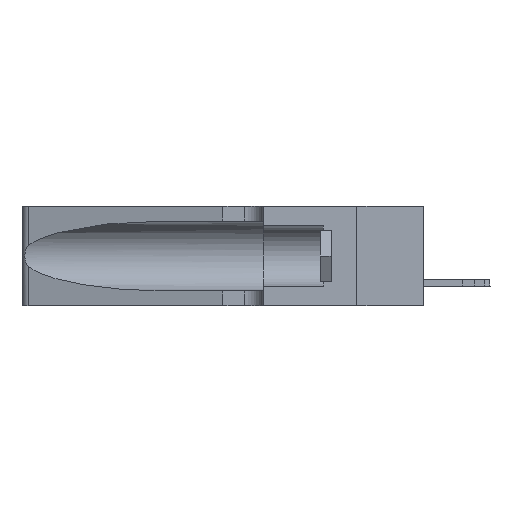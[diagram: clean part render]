
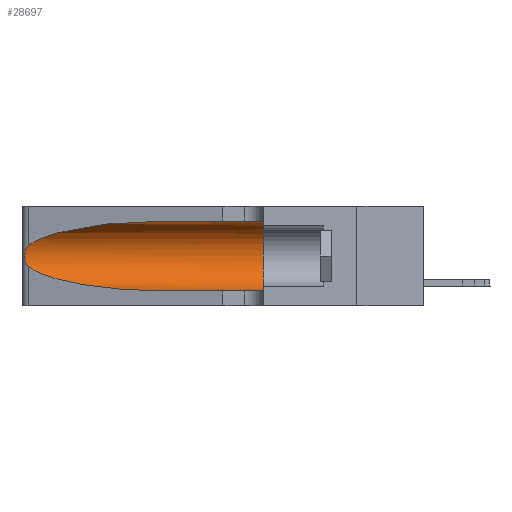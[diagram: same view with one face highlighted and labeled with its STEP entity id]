
A CAD part, left-side view. The second image highlights one B-rep face of the part: STEP entity #28697.
In plain terms, the highlighted cylindrical face has radius 3.308 mm (diameter 6.617 mm), a partial arc.
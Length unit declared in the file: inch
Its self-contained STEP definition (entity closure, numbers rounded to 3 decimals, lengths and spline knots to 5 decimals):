
#554 =( BOUNDED_CURVE ( )  B_SPLINE_CURVE ( 3, ( #15798, #22592, #4227, #18102 ),
 .UNSPECIFIED., .F., .T. ) 
 B_SPLINE_CURVE_WITH_KNOTS ( ( 4, 4 ),
 ( 3.44316, 4.71239 ),
 .UNSPECIFIED. ) 
 CURVE ( )  GEOMETRIC_REPRESENTATION_ITEM ( )  RATIONAL_B_SPLINE_CURVE ( ( 1., 0.87, 0.87, 1. ) ) 
 REPRESENTATION_ITEM ( '' )  );
#1014 = AXIS2_PLACEMENT_3D ( 'NONE', #15501, #12953, #17614 ) ;
#1427 = EDGE_LOOP ( 'NONE', ( #17655, #5297, #15512, #22694, #8040, #17215 ) ) ;
#1759 = CARTESIAN_POINT ( 'NONE',  ( 0.25639, 1.23184, 0.21858 ) ) ;
#2058 = VERTEX_POINT ( 'NONE', #29557 ) ;
#2132 = CARTESIAN_POINT ( 'NONE',  ( 0.1305, 0.72297, 0.31525 ) ) ;
#2255 = CARTESIAN_POINT ( 'NONE',  ( 0.1305, 0.72297, 0.31525 ) ) ;
#2358 = CARTESIAN_POINT ( 'NONE',  ( 0.18966, 0.96281, 0.31525 ) ) ;
#3695 = CARTESIAN_POINT ( 'NONE',  ( 0.25856, 1.23593, 0.16098 ) ) ;
#3727 = VERTEX_POINT ( 'NONE', #7228 ) ;
#3909 = CARTESIAN_POINT ( 'NONE',  ( 0.25787, 1.23484, 0.2124 ) ) ;
#3962 = VERTEX_POINT ( 'NONE', #2132 ) ;
#4227 = CARTESIAN_POINT ( 'NONE',  ( 0.18966, 0.96281, 0.05475 ) ) ;
#4810 = EDGE_CURVE ( 'NONE', #20243, #8025, #29675, .T. ) ;
#5297 = ORIENTED_EDGE ( 'NONE', *, *, #4810, .T. ) ;
#6136 = CARTESIAN_POINT ( 'NONE',  ( 0.25854, 1.2359, 0.20912 ) ) ;
#6489 = LINE ( 'NONE', #26555, #17339 ) ;
#6743 = CARTESIAN_POINT ( 'NONE',  ( 0.25487, 1.22718, 0.22369 ) ) ;
#7044 = EDGE_CURVE ( 'NONE', #26995, #2058, #26126, .T. ) ;
#7228 = CARTESIAN_POINT ( 'NONE',  ( 0.1305, 0.72297, 0.05475 ) ) ;
#8025 = VERTEX_POINT ( 'NONE', #8267 ) ;
#8040 = ORIENTED_EDGE ( 'NONE', *, *, #7044, .F. ) ;
#8267 = CARTESIAN_POINT ( 'NONE',  ( 0.25487, 1.22718, 0.14631 ) ) ;
#8480 = DIRECTION ( 'NONE',  ( 0., -1., 0. ) ) ;
#8678 = CARTESIAN_POINT ( 'NONE',  ( 0.25487, 1.22718, 0.22369 ) ) ;
#8778 = CARTESIAN_POINT ( 'NONE',  ( 0.25555, 1.22994, 0.2215 ) ) ;
#8940 = EDGE_CURVE ( 'NONE', #3727, #2058, #6489, .T. ) ;
#10435 = DIRECTION ( 'NONE',  ( 0., -1., 0. ) ) ;
#10907 = CARTESIAN_POINT ( 'NONE',  ( 0.25555, 1.22993, 0.14849 ) ) ;
#11491 = CARTESIAN_POINT ( 'NONE',  ( 0.2373, 1.15595, 0.28018 ) ) ;
#12953 = DIRECTION ( 'NONE',  ( 0., 1., 0. ) ) ;
#13348 = CARTESIAN_POINT ( 'NONE',  ( 0.26018, 1.23835, 0.19895 ) ) ;
#14706 = VECTOR ( 'NONE', #23115, 39.37008 ) ;
#14873 = CARTESIAN_POINT ( 'NONE',  ( 0.1305, 0.35, 0.31525 ) ) ;
#14885 = FACE_OUTER_BOUND ( 'NONE', #1427, .T. ) ;
#15263 = CARTESIAN_POINT ( 'NONE',  ( 0.26075, 1.23896, 0.19203 ) ) ;
#15384 = CARTESIAN_POINT ( 'NONE',  ( 0.1305, 1.61858, 0.31525 ) ) ;
#15501 = CARTESIAN_POINT ( 'NONE',  ( 0.1305, 0.35, 0.185 ) ) ;
#15512 = ORIENTED_EDGE ( 'NONE', *, *, #24012, .T. ) ;
#15798 = CARTESIAN_POINT ( 'NONE',  ( 0.25487, 1.22718, 0.14631 ) ) ;
#16136 = AXIS2_PLACEMENT_3D ( 'NONE', #26480, #10435, #26568 ) ;
#16374 = CYLINDRICAL_SURFACE ( 'NONE', #16136, 0.13025 ) ;
#17215 = ORIENTED_EDGE ( 'NONE', *, *, #26096, .F. ) ;
#17339 = VECTOR ( 'NONE', #8480, 39.37008 ) ;
#17614 = DIRECTION ( 'NONE',  ( 0., 0., 1. ) ) ;
#17655 = ORIENTED_EDGE ( 'NONE', *, *, #19843, .T. ) ;
#18102 = CARTESIAN_POINT ( 'NONE',  ( 0.1305, 0.72297, 0.05475 ) ) ;
#19812 =( BOUNDED_CURVE ( )  B_SPLINE_CURVE ( 3, ( #2255, #2358, #11491, #6743 ),
 .UNSPECIFIED., .F., .T. ) 
 B_SPLINE_CURVE_WITH_KNOTS ( ( 4, 4 ),
 ( 1.5708, 2.84003 ),
 .UNSPECIFIED. ) 
 CURVE ( )  GEOMETRIC_REPRESENTATION_ITEM ( )  RATIONAL_B_SPLINE_CURVE ( ( 1., 0.87, 0.87, 1. ) ) 
 REPRESENTATION_ITEM ( '' )  );
#19843 = EDGE_CURVE ( 'NONE', #3962, #20243, #19812, .T. ) ;
#20191 = CARTESIAN_POINT ( 'NONE',  ( 0.25487, 1.22718, 0.14631 ) ) ;
#20243 = VERTEX_POINT ( 'NONE', #22446 ) ;
#20859 = LINE ( 'NONE', #15384, #14706 ) ;
#22273 = CARTESIAN_POINT ( 'NONE',  ( 0.26075, 1.23896, 0.178 ) ) ;
#22446 = CARTESIAN_POINT ( 'NONE',  ( 0.25487, 1.22718, 0.22369 ) ) ;
#22592 = CARTESIAN_POINT ( 'NONE',  ( 0.2373, 1.15595, 0.08982 ) ) ;
#22694 = ORIENTED_EDGE ( 'NONE', *, *, #8940, .T. ) ;
#23115 = DIRECTION ( 'NONE',  ( 0., -1., 0. ) ) ;
#24012 = EDGE_CURVE ( 'NONE', #8025, #3727, #554, .T. ) ;
#24841 = CARTESIAN_POINT ( 'NONE',  ( 0.25639, 1.23186, 0.15144 ) ) ;
#26096 = EDGE_CURVE ( 'NONE', #3962, #26995, #20859, .T. ) ;
#26126 = CIRCLE ( 'NONE', #1014, 0.13025 ) ;
#26480 = CARTESIAN_POINT ( 'NONE',  ( 0.1305, 1.61858, 0.185 ) ) ;
#26555 = CARTESIAN_POINT ( 'NONE',  ( 0.1305, 1.61858, 0.05475 ) ) ;
#26568 = DIRECTION ( 'NONE',  ( 0., 0., -1. ) ) ;
#26995 = VERTEX_POINT ( 'NONE', #14873 ) ;
#28697 = ADVANCED_FACE ( 'NONE', ( #14885 ), #16374, .F. ) ;
#29307 = CARTESIAN_POINT ( 'NONE',  ( 0.25789, 1.23486, 0.15765 ) ) ;
#29427 = CARTESIAN_POINT ( 'NONE',  ( 0.26017, 1.23833, 0.17102 ) ) ;
#29557 = CARTESIAN_POINT ( 'NONE',  ( 0.1305, 0.35, 0.05475 ) ) ;
#29675 = B_SPLINE_CURVE_WITH_KNOTS ( 'NONE', 3,
 ( #8678, #8778, #1759, #3909, #6136, #13348, #15263, #22273, #29427, #3695, #29307, #24841, #10907, #20191 ),
 .UNSPECIFIED., .F., .F.,
 ( 4, 2, 2, 2, 2, 2, 4 ),
 ( 0., 0.00027, 0.00053, 0.00107, 0.0016, 0.00187, 0.00214 ),
 .UNSPECIFIED. ) ;
